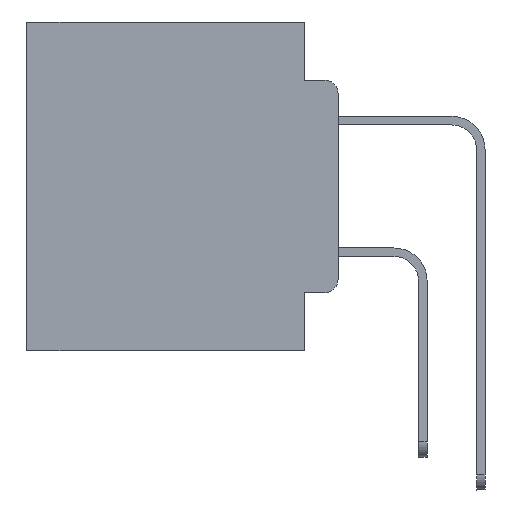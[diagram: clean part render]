
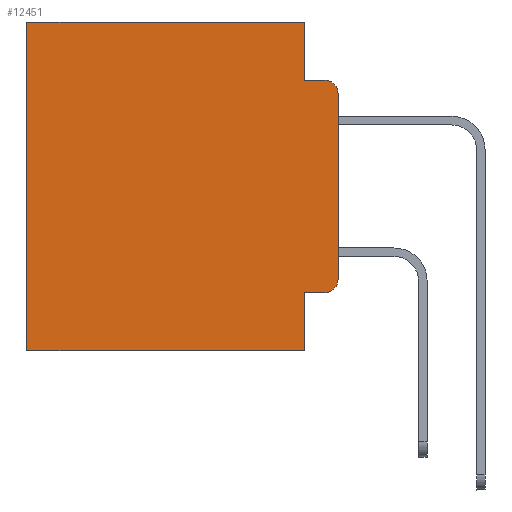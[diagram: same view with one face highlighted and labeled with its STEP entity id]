
A CAD part, left-side view. The second image highlights one B-rep face of the part: STEP entity #12451.
In plain terms, the highlighted planar face has unit normal (-1, 0, 0).
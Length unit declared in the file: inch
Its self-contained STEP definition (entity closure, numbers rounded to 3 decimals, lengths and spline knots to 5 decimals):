
#1033 = EDGE_CURVE ( 'NONE', #20590, #9534, #27901, .T. ) ;
#1066 = VERTEX_POINT ( 'NONE', #9475 ) ;
#1492 = VECTOR ( 'NONE', #22726, 39.37008 ) ;
#1615 = DIRECTION ( 'NONE',  ( 0., 0., -1. ) ) ;
#1678 = DIRECTION ( 'NONE',  ( 0., -1., 0. ) ) ;
#1838 = CARTESIAN_POINT ( 'NONE',  ( 0.298, 0.051, 0. ) ) ;
#2052 = ORIENTED_EDGE ( 'NONE', *, *, #2959, .T. ) ;
#2912 = DIRECTION ( 'NONE',  ( 0., -1., 0. ) ) ;
#2919 = EDGE_CURVE ( 'NONE', #26097, #15472, #11757, .T. ) ;
#2959 = EDGE_CURVE ( 'NONE', #26097, #1066, #18512, .T. ) ;
#3260 = ORIENTED_EDGE ( 'NONE', *, *, #27647, .T. ) ;
#3420 = VECTOR ( 'NONE', #11511, 39.37008 ) ;
#3610 = CARTESIAN_POINT ( 'NONE',  ( 0.298, 0., 0. ) ) ;
#3727 = DIRECTION ( 'NONE',  ( 0., 1., 0. ) ) ;
#4353 = ORIENTED_EDGE ( 'NONE', *, *, #16345, .F. ) ;
#5513 = VECTOR ( 'NONE', #14039, 39.37008 ) ;
#5535 = ORIENTED_EDGE ( 'NONE', *, *, #2919, .F. ) ;
#5670 = ORIENTED_EDGE ( 'NONE', *, *, #24240, .F. ) ;
#5885 = VERTEX_POINT ( 'NONE', #11389 ) ;
#6319 = DIRECTION ( 'NONE',  ( 1., 0., 0. ) ) ;
#6736 = CARTESIAN_POINT ( 'NONE',  ( 0.298, 0.051, 0. ) ) ;
#7142 = LINE ( 'NONE', #22476, #3420 ) ;
#8148 = LINE ( 'NONE', #16972, #11128 ) ;
#8212 = FACE_OUTER_BOUND ( 'NONE', #21189, .T. ) ;
#8220 = LINE ( 'NONE', #1838, #11933 ) ;
#8367 = DIRECTION ( 'NONE',  ( 0., 0., -1. ) ) ;
#9475 = CARTESIAN_POINT ( 'NONE',  ( 0.298, 0.02, -0.4115 ) ) ;
#9534 = VERTEX_POINT ( 'NONE', #13650 ) ;
#9550 = EDGE_CURVE ( 'NONE', #20590, #15606, #7142, .T. ) ;
#9901 = DIRECTION ( 'NONE',  ( -1., 0., 0. ) ) ;
#10042 = CARTESIAN_POINT ( 'NONE',  ( 0.298, 0.02, -0.1085 ) ) ;
#10905 = AXIS2_PLACEMENT_3D ( 'NONE', #19601, #6319, #13115 ) ;
#11128 = VECTOR ( 'NONE', #1615, 39.37008 ) ;
#11389 = CARTESIAN_POINT ( 'NONE',  ( 0.298, 0.473, 0. ) ) ;
#11511 = DIRECTION ( 'NONE',  ( 0., 0., -1. ) ) ;
#11757 = LINE ( 'NONE', #27217, #1492 ) ;
#11933 = VECTOR ( 'NONE', #8367, 39.37008 ) ;
#12451 = ADVANCED_FACE ( 'NONE', ( #8212 ), #14986, .F. ) ;
#12686 = LINE ( 'NONE', #21499, #25358 ) ;
#13115 = DIRECTION ( 'NONE',  ( 0., 0., -1. ) ) ;
#13549 = ORIENTED_EDGE ( 'NONE', *, *, #24200, .F. ) ;
#13650 = CARTESIAN_POINT ( 'NONE',  ( 0.298, 0.02, -0.0885 ) ) ;
#14039 = DIRECTION ( 'NONE',  ( 0., 1., 0. ) ) ;
#14300 = EDGE_CURVE ( 'NONE', #1066, #15606, #26677, .T. ) ;
#14986 = PLANE ( 'NONE',  #10905 ) ;
#15260 = ORIENTED_EDGE ( 'NONE', *, *, #28567, .T. ) ;
#15289 = LINE ( 'NONE', #19607, #16509 ) ;
#15472 = VERTEX_POINT ( 'NONE', #17828 ) ;
#15606 = VERTEX_POINT ( 'NONE', #20287 ) ;
#15792 = CARTESIAN_POINT ( 'NONE',  ( 0.298, 0.051, -0.4115 ) ) ;
#16052 = CARTESIAN_POINT ( 'NONE',  ( 0.298, 0.473, -0.5 ) ) ;
#16345 = EDGE_CURVE ( 'NONE', #19675, #9534, #12686, .T. ) ;
#16447 = VERTEX_POINT ( 'NONE', #6736 ) ;
#16509 = VECTOR ( 'NONE', #3727, 39.37008 ) ;
#16972 = CARTESIAN_POINT ( 'NONE',  ( 0.298, 0.473, 0. ) ) ;
#17196 = ORIENTED_EDGE ( 'NONE', *, *, #9550, .F. ) ;
#17548 = CARTESIAN_POINT ( 'NONE',  ( 0.298, 0., -0.1085 ) ) ;
#17828 = CARTESIAN_POINT ( 'NONE',  ( 0.298, 0.051, -0.5 ) ) ;
#17988 = VERTEX_POINT ( 'NONE', #16052 ) ;
#18512 = LINE ( 'NONE', #15792, #24573 ) ;
#18773 = DIRECTION ( 'NONE',  ( -1., 0., 0. ) ) ;
#19601 = CARTESIAN_POINT ( 'NONE',  ( 0.298, 0., 0. ) ) ;
#19607 = CARTESIAN_POINT ( 'NONE',  ( 0.298, 0., -0.5 ) ) ;
#19675 = VERTEX_POINT ( 'NONE', #26719 ) ;
#20287 = CARTESIAN_POINT ( 'NONE',  ( 0.298, 0., -0.3915 ) ) ;
#20525 = AXIS2_PLACEMENT_3D ( 'NONE', #10042, #9901, #27671 ) ;
#20590 = VERTEX_POINT ( 'NONE', #17548 ) ;
#20673 = CARTESIAN_POINT ( 'NONE',  ( 0.298, 0.02, -0.3915 ) ) ;
#21189 = EDGE_LOOP ( 'NONE', ( #17196, #23026, #4353, #13549, #3260, #15260, #5670, #5535, #2052, #26112 ) ) ;
#21499 = CARTESIAN_POINT ( 'NONE',  ( 0.298, 0.051, -0.0885 ) ) ;
#22476 = CARTESIAN_POINT ( 'NONE',  ( 0.298, 0., 0. ) ) ;
#22726 = DIRECTION ( 'NONE',  ( 0., 0., -1. ) ) ;
#23026 = ORIENTED_EDGE ( 'NONE', *, *, #1033, .T. ) ;
#23412 = LINE ( 'NONE', #3610, #5513 ) ;
#24200 = EDGE_CURVE ( 'NONE', #16447, #19675, #8220, .T. ) ;
#24209 = CARTESIAN_POINT ( 'NONE',  ( 0.298, 0.051, -0.4115 ) ) ;
#24240 = EDGE_CURVE ( 'NONE', #15472, #17988, #15289, .T. ) ;
#24573 = VECTOR ( 'NONE', #2912, 39.37008 ) ;
#25006 = DIRECTION ( 'NONE',  ( 0., 0., -1. ) ) ;
#25358 = VECTOR ( 'NONE', #1678, 39.37008 ) ;
#26097 = VERTEX_POINT ( 'NONE', #24209 ) ;
#26112 = ORIENTED_EDGE ( 'NONE', *, *, #14300, .T. ) ;
#26677 = CIRCLE ( 'NONE', #27582, 0.02 ) ;
#26719 = CARTESIAN_POINT ( 'NONE',  ( 0.298, 0.051, -0.0885 ) ) ;
#27217 = CARTESIAN_POINT ( 'NONE',  ( 0.298, 0.051, 0. ) ) ;
#27582 = AXIS2_PLACEMENT_3D ( 'NONE', #20673, #18773, #25006 ) ;
#27647 = EDGE_CURVE ( 'NONE', #16447, #5885, #23412, .T. ) ;
#27671 = DIRECTION ( 'NONE',  ( 0., 0., -1. ) ) ;
#27901 = CIRCLE ( 'NONE', #20525, 0.02 ) ;
#28567 = EDGE_CURVE ( 'NONE', #5885, #17988, #8148, .T. ) ;
